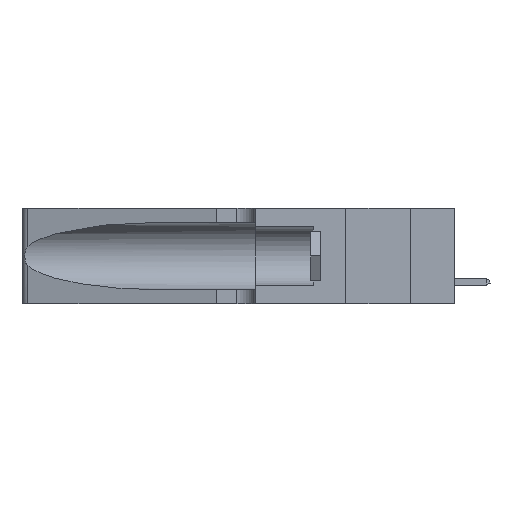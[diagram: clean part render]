
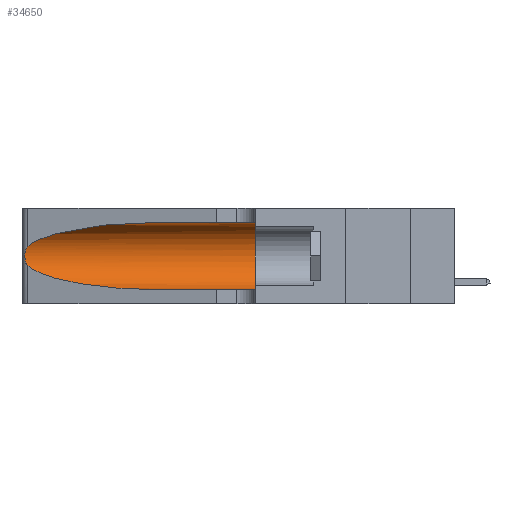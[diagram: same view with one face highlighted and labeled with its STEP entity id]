
A CAD part, left-side view. The second image highlights one B-rep face of the part: STEP entity #34650.
In plain terms, the highlighted cylindrical face has radius 3.308 mm (diameter 6.617 mm), a partial arc.
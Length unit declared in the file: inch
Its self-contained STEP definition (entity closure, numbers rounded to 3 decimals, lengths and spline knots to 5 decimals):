
#26 = LINE ( 'NONE', #16017, #36393 ) ;
#387 = EDGE_CURVE ( 'NONE', #32605, #19681, #39903, .T. ) ;
#654 = EDGE_CURVE ( 'NONE', #35316, #7989, #2436, .T. ) ;
#1388 = VERTEX_POINT ( 'NONE', #21184 ) ;
#1519 = CARTESIAN_POINT ( 'NONE',  ( 0.25555, 1.22993, 0.14849 ) ) ;
#2436 = CIRCLE ( 'NONE', #26831, 0.13025 ) ;
#3414 = ORIENTED_EDGE ( 'NONE', *, *, #387, .T. ) ;
#3511 = CARTESIAN_POINT ( 'NONE',  ( 0.25856, 1.23593, 0.16098 ) ) ;
#4017 = CARTESIAN_POINT ( 'NONE',  ( 0.1305, 1.61858, 0.05475 ) ) ;
#4204 = EDGE_CURVE ( 'NONE', #19681, #7989, #31672, .T. ) ;
#4550 = EDGE_CURVE ( 'NONE', #1388, #18183, #23610, .T. ) ;
#7018 = CARTESIAN_POINT ( 'NONE',  ( 0.1305, 1.61858, 0.185 ) ) ;
#7209 = ORIENTED_EDGE ( 'NONE', *, *, #37459, .F. ) ;
#7806 = CARTESIAN_POINT ( 'NONE',  ( 0.25639, 1.23186, 0.15144 ) ) ;
#7989 = VERTEX_POINT ( 'NONE', #8557 ) ;
#8557 = CARTESIAN_POINT ( 'NONE',  ( 0.1305, 0.35, 0.05475 ) ) ;
#8574 = CARTESIAN_POINT ( 'NONE',  ( 0.1305, 0.72297, 0.05475 ) ) ;
#8592 = DIRECTION ( 'NONE',  ( 0., 0., 1. ) ) ;
#9100 = CYLINDRICAL_SURFACE ( 'NONE', #36318, 0.13025 ) ;
#10418 = DIRECTION ( 'NONE',  ( 0., 0., -1. ) ) ;
#10490 = CARTESIAN_POINT ( 'NONE',  ( 0.25639, 1.23184, 0.21858 ) ) ;
#10570 = DIRECTION ( 'NONE',  ( 0., -1., 0. ) ) ;
#11737 = VECTOR ( 'NONE', #18757, 39.37008 ) ;
#12458 = CARTESIAN_POINT ( 'NONE',  ( 0.25487, 1.22718, 0.22369 ) ) ;
#13477 = CARTESIAN_POINT ( 'NONE',  ( 0.25787, 1.23484, 0.2124 ) ) ;
#16017 = CARTESIAN_POINT ( 'NONE',  ( 0.1305, 1.61858, 0.31525 ) ) ;
#16064 = CARTESIAN_POINT ( 'NONE',  ( 0.1305, 0.72297, 0.05475 ) ) ;
#16824 = CARTESIAN_POINT ( 'NONE',  ( 0.2373, 1.15595, 0.28018 ) ) ;
#17574 = CARTESIAN_POINT ( 'NONE',  ( 0.26075, 1.23896, 0.19203 ) ) ;
#17601 = CARTESIAN_POINT ( 'NONE',  ( 0.1305, 0.35, 0.31525 ) ) ;
#18183 = VERTEX_POINT ( 'NONE', #37605 ) ;
#18757 = DIRECTION ( 'NONE',  ( 0., -1., 0. ) ) ;
#19681 = VERTEX_POINT ( 'NONE', #16064 ) ;
#20238 = CARTESIAN_POINT ( 'NONE',  ( 0.18966, 0.96281, 0.31525 ) ) ;
#20864 = EDGE_LOOP ( 'NONE', ( #24486, #36233, #3414, #23852, #22553, #7209 ) ) ;
#21184 = CARTESIAN_POINT ( 'NONE',  ( 0.1305, 0.72297, 0.31525 ) ) ;
#21337 = CARTESIAN_POINT ( 'NONE',  ( 0.25487, 1.22718, 0.22369 ) ) ;
#21490 = CARTESIAN_POINT ( 'NONE',  ( 0.25555, 1.22994, 0.2215 ) ) ;
#22187 = CARTESIAN_POINT ( 'NONE',  ( 0.18966, 0.96281, 0.05475 ) ) ;
#22553 = ORIENTED_EDGE ( 'NONE', *, *, #654, .F. ) ;
#23435 = CARTESIAN_POINT ( 'NONE',  ( 0.25487, 1.22718, 0.14631 ) ) ;
#23610 =( BOUNDED_CURVE ( )  B_SPLINE_CURVE ( 3, ( #34258, #20238, #16824, #12458 ),
 .UNSPECIFIED., .F., .T. ) 
 B_SPLINE_CURVE_WITH_KNOTS ( ( 4, 4 ),
 ( 1.5708, 2.84003 ),
 .UNSPECIFIED. ) 
 CURVE ( )  GEOMETRIC_REPRESENTATION_ITEM ( )  RATIONAL_B_SPLINE_CURVE ( ( 1., 0.87, 0.87, 1. ) ) 
 REPRESENTATION_ITEM ( '' )  );
#23852 = ORIENTED_EDGE ( 'NONE', *, *, #4204, .T. ) ;
#24486 = ORIENTED_EDGE ( 'NONE', *, *, #4550, .T. ) ;
#24690 = CARTESIAN_POINT ( 'NONE',  ( 0.26017, 1.23833, 0.17102 ) ) ;
#25442 = CARTESIAN_POINT ( 'NONE',  ( 0.25789, 1.23486, 0.15765 ) ) ;
#26831 = AXIS2_PLACEMENT_3D ( 'NONE', #29637, #33152, #8592 ) ;
#27764 = EDGE_CURVE ( 'NONE', #18183, #32605, #37964, .T. ) ;
#27921 = FACE_OUTER_BOUND ( 'NONE', #20864, .T. ) ;
#28987 = CARTESIAN_POINT ( 'NONE',  ( 0.25487, 1.22718, 0.14631 ) ) ;
#29637 = CARTESIAN_POINT ( 'NONE',  ( 0.1305, 0.35, 0.185 ) ) ;
#31672 = LINE ( 'NONE', #4017, #11737 ) ;
#32506 = CARTESIAN_POINT ( 'NONE',  ( 0.2373, 1.15595, 0.08982 ) ) ;
#32605 = VERTEX_POINT ( 'NONE', #23435 ) ;
#33152 = DIRECTION ( 'NONE',  ( 0., 1., 0. ) ) ;
#33164 = CARTESIAN_POINT ( 'NONE',  ( 0.25487, 1.22718, 0.14631 ) ) ;
#34258 = CARTESIAN_POINT ( 'NONE',  ( 0.1305, 0.72297, 0.31525 ) ) ;
#34650 = ADVANCED_FACE ( 'NONE', ( #27921 ), #9100, .F. ) ;
#35135 = CARTESIAN_POINT ( 'NONE',  ( 0.25854, 1.2359, 0.20912 ) ) ;
#35316 = VERTEX_POINT ( 'NONE', #17601 ) ;
#36233 = ORIENTED_EDGE ( 'NONE', *, *, #27764, .T. ) ;
#36318 = AXIS2_PLACEMENT_3D ( 'NONE', #7018, #10570, #10418 ) ;
#36393 = VECTOR ( 'NONE', #44356, 39.37008 ) ;
#37459 = EDGE_CURVE ( 'NONE', #1388, #35316, #26, .T. ) ;
#37605 = CARTESIAN_POINT ( 'NONE',  ( 0.25487, 1.22718, 0.22369 ) ) ;
#37964 = B_SPLINE_CURVE_WITH_KNOTS ( 'NONE', 3,
 ( #21337, #21490, #10490, #13477, #35135, #38680, #17574, #42204, #24690, #3511, #25442, #7806, #1519, #33164 ),
 .UNSPECIFIED., .F., .F.,
 ( 4, 2, 2, 2, 2, 2, 4 ),
 ( 0., 0.00027, 0.00053, 0.00107, 0.0016, 0.00187, 0.00214 ),
 .UNSPECIFIED. ) ;
#38680 = CARTESIAN_POINT ( 'NONE',  ( 0.26018, 1.23835, 0.19895 ) ) ;
#39903 =( BOUNDED_CURVE ( )  B_SPLINE_CURVE ( 3, ( #28987, #32506, #22187, #8574 ),
 .UNSPECIFIED., .F., .F. ) 
 B_SPLINE_CURVE_WITH_KNOTS ( ( 4, 4 ),
 ( 3.44316, 4.71239 ),
 .UNSPECIFIED. ) 
 CURVE ( )  GEOMETRIC_REPRESENTATION_ITEM ( )  RATIONAL_B_SPLINE_CURVE ( ( 1., 0.87, 0.87, 1. ) ) 
 REPRESENTATION_ITEM ( '' )  );
#42204 = CARTESIAN_POINT ( 'NONE',  ( 0.26075, 1.23896, 0.178 ) ) ;
#44356 = DIRECTION ( 'NONE',  ( 0., -1., 0. ) ) ;
